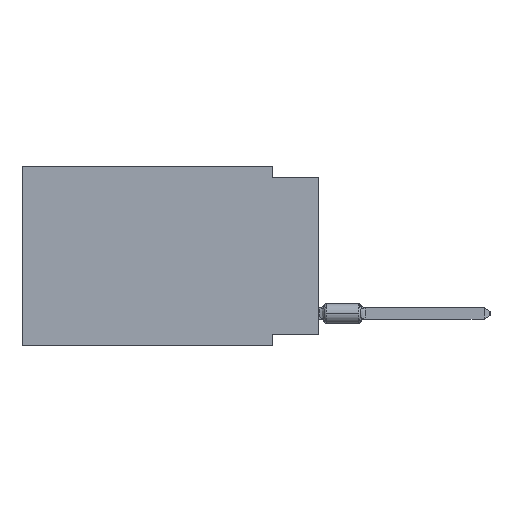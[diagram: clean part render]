
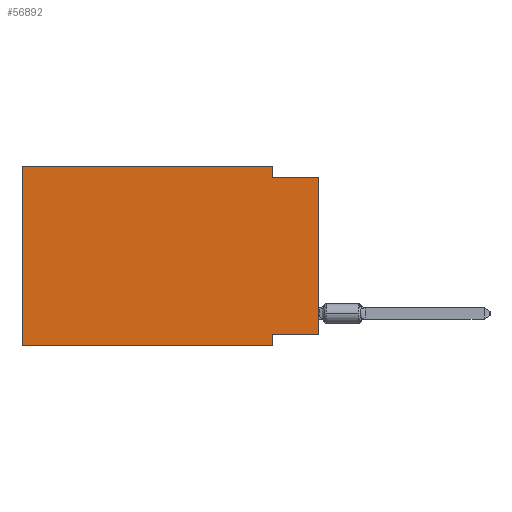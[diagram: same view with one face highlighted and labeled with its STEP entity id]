
A CAD part, left-side view. The second image highlights one B-rep face of the part: STEP entity #56892.
In plain terms, the highlighted planar face has unit normal (-1, 0, 0).
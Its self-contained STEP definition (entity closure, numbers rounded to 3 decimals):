
#1824 = EDGE_LOOP ( 'NONE', ( #43420, #47891, #15078, #38016, #61791, #61527, #8958, #34381 ) ) ;
#3668 = VERTEX_POINT ( 'NONE', #62271 ) ;
#4520 = DIRECTION ( 'NONE',  ( 0., 0., -1. ) ) ;
#4736 = CARTESIAN_POINT ( 'NONE',  ( 0., 2.54, -9.271 ) ) ;
#5240 = LINE ( 'NONE', #40770, #59782 ) ;
#5710 = LINE ( 'NONE', #25867, #12820 ) ;
#7992 = CARTESIAN_POINT ( 'NONE',  ( 0., 2.54, 0. ) ) ;
#8126 = EDGE_CURVE ( 'NONE', #3668, #34913, #5710, .T. ) ;
#8958 = ORIENTED_EDGE ( 'NONE', *, *, #61258, .F. ) ;
#12820 = VECTOR ( 'NONE', #67561, 1000. ) ;
#14976 = VERTEX_POINT ( 'NONE', #44367 ) ;
#15078 = ORIENTED_EDGE ( 'NONE', *, *, #17448, .F. ) ;
#15111 = CARTESIAN_POINT ( 'NONE',  ( 0., 2.54, 0. ) ) ;
#16455 = LINE ( 'NONE', #15111, #34077 ) ;
#16746 = VECTOR ( 'NONE', #48875, 1000. ) ;
#17448 = EDGE_CURVE ( 'NONE', #48929, #64136, #16455, .T. ) ;
#18138 = EDGE_CURVE ( 'NONE', #14976, #48929, #47368, .T. ) ;
#18845 = LINE ( 'NONE', #39693, #37095 ) ;
#19534 = LINE ( 'NONE', #56094, #54891 ) ;
#19536 = DIRECTION ( 'NONE',  ( 1., 0., 0. ) ) ;
#20424 = CARTESIAN_POINT ( 'NONE',  ( 0., 16.383, -9.906 ) ) ;
#21280 = DIRECTION ( 'NONE',  ( 0., -1., 0. ) ) ;
#24330 = PLANE ( 'NONE',  #42344 ) ;
#24663 = FACE_OUTER_BOUND ( 'NONE', #1824, .T. ) ;
#24787 = CARTESIAN_POINT ( 'NONE',  ( 0., 2.54, -9.906 ) ) ;
#25867 = CARTESIAN_POINT ( 'NONE',  ( 0., 0., -9.271 ) ) ;
#28660 = VECTOR ( 'NONE', #58294, 1000. ) ;
#29792 = DIRECTION ( 'NONE',  ( 0., 0., 1. ) ) ;
#29930 = DIRECTION ( 'NONE',  ( 0., 0., -1. ) ) ;
#30933 = LINE ( 'NONE', #24787, #67272 ) ;
#32630 = VERTEX_POINT ( 'NONE', #62474 ) ;
#34077 = VECTOR ( 'NONE', #37278, 1000. ) ;
#34381 = ORIENTED_EDGE ( 'NONE', *, *, #8126, .F. ) ;
#34913 = VERTEX_POINT ( 'NONE', #4736 ) ;
#37095 = VECTOR ( 'NONE', #41037, 1000. ) ;
#37278 = DIRECTION ( 'NONE',  ( 0., 0., -1. ) ) ;
#37782 = CARTESIAN_POINT ( 'NONE',  ( 0., 16.383, 0. ) ) ;
#38016 = ORIENTED_EDGE ( 'NONE', *, *, #18138, .F. ) ;
#39502 = EDGE_CURVE ( 'NONE', #64136, #32630, #5240, .T. ) ;
#39693 = CARTESIAN_POINT ( 'NONE',  ( 0., 16.383, -9.906 ) ) ;
#40770 = CARTESIAN_POINT ( 'NONE',  ( 0., 0., -0.635 ) ) ;
#41037 = DIRECTION ( 'NONE',  ( 0., -1., 0. ) ) ;
#41743 = VERTEX_POINT ( 'NONE', #20424 ) ;
#42344 = AXIS2_PLACEMENT_3D ( 'NONE', #60876, #19536, #4520 ) ;
#42589 = CARTESIAN_POINT ( 'NONE',  ( 0., 2.54, -9.906 ) ) ;
#43420 = ORIENTED_EDGE ( 'NONE', *, *, #53105, .T. ) ;
#43651 = EDGE_CURVE ( 'NONE', #41743, #47537, #18845, .T. ) ;
#44367 = CARTESIAN_POINT ( 'NONE',  ( 0., 16.383, 0. ) ) ;
#47368 = LINE ( 'NONE', #37782, #28660 ) ;
#47537 = VERTEX_POINT ( 'NONE', #42589 ) ;
#47891 = ORIENTED_EDGE ( 'NONE', *, *, #39502, .F. ) ;
#48875 = DIRECTION ( 'NONE',  ( 0., 0., 1. ) ) ;
#48929 = VERTEX_POINT ( 'NONE', #7992 ) ;
#51071 = EDGE_CURVE ( 'NONE', #41743, #14976, #19534, .T. ) ;
#53105 = EDGE_CURVE ( 'NONE', #3668, #32630, #65626, .T. ) ;
#54891 = VECTOR ( 'NONE', #29792, 1000. ) ;
#56094 = CARTESIAN_POINT ( 'NONE',  ( 0., 16.383, 0. ) ) ;
#56892 = ADVANCED_FACE ( 'NONE', ( #24663 ), #24330, .F. ) ;
#58294 = DIRECTION ( 'NONE',  ( 0., -1., 0. ) ) ;
#59782 = VECTOR ( 'NONE', #21280, 1000. ) ;
#60478 = CARTESIAN_POINT ( 'NONE',  ( 0., 0., 0. ) ) ;
#60876 = CARTESIAN_POINT ( 'NONE',  ( 0., 16.383, 0. ) ) ;
#61258 = EDGE_CURVE ( 'NONE', #34913, #47537, #30933, .T. ) ;
#61527 = ORIENTED_EDGE ( 'NONE', *, *, #43651, .T. ) ;
#61791 = ORIENTED_EDGE ( 'NONE', *, *, #51071, .F. ) ;
#62271 = CARTESIAN_POINT ( 'NONE',  ( 0., 0., -9.271 ) ) ;
#62474 = CARTESIAN_POINT ( 'NONE',  ( 0., 0., -0.635 ) ) ;
#63965 = CARTESIAN_POINT ( 'NONE',  ( 0., 2.54, -0.635 ) ) ;
#64136 = VERTEX_POINT ( 'NONE', #63965 ) ;
#65626 = LINE ( 'NONE', #60478, #16746 ) ;
#67272 = VECTOR ( 'NONE', #29930, 1000. ) ;
#67561 = DIRECTION ( 'NONE',  ( 0., 1., 0. ) ) ;
